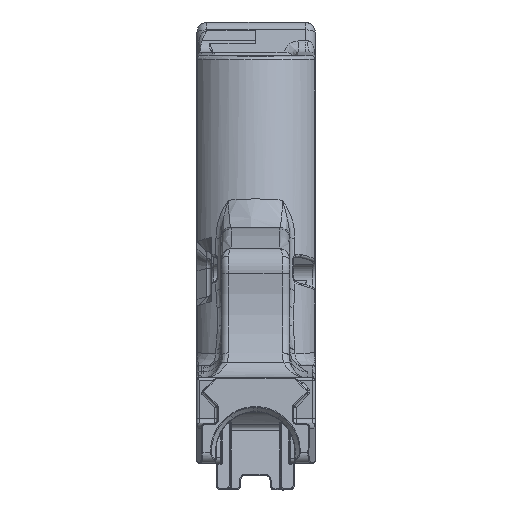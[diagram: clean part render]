
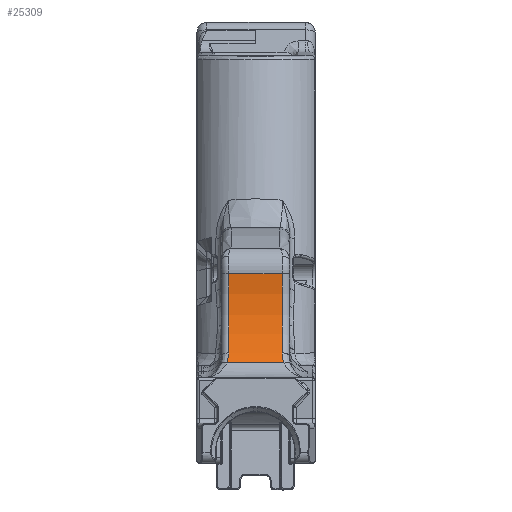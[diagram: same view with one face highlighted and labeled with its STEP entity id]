
A CAD part, left-side view. The second image highlights one B-rep face of the part: STEP entity #25309.
In plain terms, the highlighted cylindrical face has radius 27 mm (diameter 54 mm), a partial arc.
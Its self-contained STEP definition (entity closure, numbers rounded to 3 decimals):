
#1305=CYLINDRICAL_SURFACE('',#28051,27.);
#2494=FACE_OUTER_BOUND('',#4001,.T.);
#4001=EDGE_LOOP('',(#22220,#22221,#22222,#22223,#22224,#22225));
#5529=LINE('',#58954,#6794);
#5530=LINE('',#58956,#6795);
#6794=VECTOR('',#34396,1000.);
#6795=VECTOR('',#34399,1000.);
#7723=B_SPLINE_CURVE_WITH_KNOTS('',3,(#58471,#58472,#58473,#58474),
 .UNSPECIFIED.,.F.,.F.,(4,4),(0.,1.),.UNSPECIFIED.);
#7735=B_SPLINE_CURVE_WITH_KNOTS('',3,(#58947,#58948,#58949,#58950),
 .UNSPECIFIED.,.F.,.F.,(4,4),(0.,1.),.UNSPECIFIED.);
#8852=CIRCLE('',#28052,27.);
#8853=CIRCLE('',#28053,27.);
#11929=VERTEX_POINT('',#58457);
#11932=VERTEX_POINT('',#58465);
#11938=VERTEX_POINT('',#58945);
#11939=VERTEX_POINT('',#58946);
#11940=VERTEX_POINT('',#58951);
#11941=VERTEX_POINT('',#58953);
#15613=EDGE_CURVE('',#11932,#11929,#7723,.T.);
#15643=EDGE_CURVE('',#11938,#11939,#7735,.T.);
#15644=EDGE_CURVE('',#11940,#11938,#8852,.T.);
#15645=EDGE_CURVE('',#11940,#11941,#5529,.T.);
#15646=EDGE_CURVE('',#11929,#11941,#8853,.T.);
#15647=EDGE_CURVE('',#11939,#11932,#5530,.T.);
#22220=ORIENTED_EDGE('',*,*,#15643,.F.);
#22221=ORIENTED_EDGE('',*,*,#15644,.F.);
#22222=ORIENTED_EDGE('',*,*,#15645,.T.);
#22223=ORIENTED_EDGE('',*,*,#15646,.F.);
#22224=ORIENTED_EDGE('',*,*,#15613,.F.);
#22225=ORIENTED_EDGE('',*,*,#15647,.F.);
#25309=ADVANCED_FACE('',(#2494),#1305,.F.);
#28051=AXIS2_PLACEMENT_3D('',#58944,#34392,#34393);
#28052=AXIS2_PLACEMENT_3D('',#58952,#34394,#34395);
#28053=AXIS2_PLACEMENT_3D('',#58955,#34397,#34398);
#34392=DIRECTION('center_axis',(0.,1.,0.));
#34393=DIRECTION('ref_axis',(0.993,0.,0.119));
#34394=DIRECTION('center_axis',(0.,1.,0.));
#34395=DIRECTION('ref_axis',(0.977,0.,-0.213));
#34396=DIRECTION('',(0.,1.,0.));
#34397=DIRECTION('center_axis',(0.,-1.,0.));
#34398=DIRECTION('ref_axis',(0.977,0.,-0.213));
#34399=DIRECTION('',(0.,1.,0.));
#58457=CARTESIAN_POINT('',(-35.966,5.5,-14.895));
#58465=CARTESIAN_POINT('',(-37.185,5.854,-16.898));
#58471=CARTESIAN_POINT('Ctrl Pts',(-37.185,5.854,-16.898));
#58472=CARTESIAN_POINT('Ctrl Pts',(-36.762,5.621,-16.265));
#58473=CARTESIAN_POINT('Ctrl Pts',(-36.348,5.5,-15.589));
#58474=CARTESIAN_POINT('Ctrl Pts',(-35.966,5.5,-14.895));
#58944=CARTESIAN_POINT('Origin',(-59.613,-7.,-1.864));
#58945=CARTESIAN_POINT('',(-35.966,-5.5,-14.895));
#58946=CARTESIAN_POINT('',(-37.185,-5.854,-16.898));
#58947=CARTESIAN_POINT('Ctrl Pts',(-35.966,-5.5,-14.895));
#58948=CARTESIAN_POINT('Ctrl Pts',(-36.348,-5.5,-15.589));
#58949=CARTESIAN_POINT('Ctrl Pts',(-36.762,-5.621,
-16.265));
#58950=CARTESIAN_POINT('Ctrl Pts',(-37.185,-5.854,
-16.898));
#58951=CARTESIAN_POINT('',(-32.805,-5.5,1.354));
#58952=CARTESIAN_POINT('Origin',(-59.613,-5.5,-1.864));
#58953=CARTESIAN_POINT('',(-32.805,5.5,1.354));
#58954=CARTESIAN_POINT('',(-32.805,-7.,1.354));
#58955=CARTESIAN_POINT('Origin',(-59.613,5.5,-1.864));
#58956=CARTESIAN_POINT('',(-37.185,-7.,-16.898));
